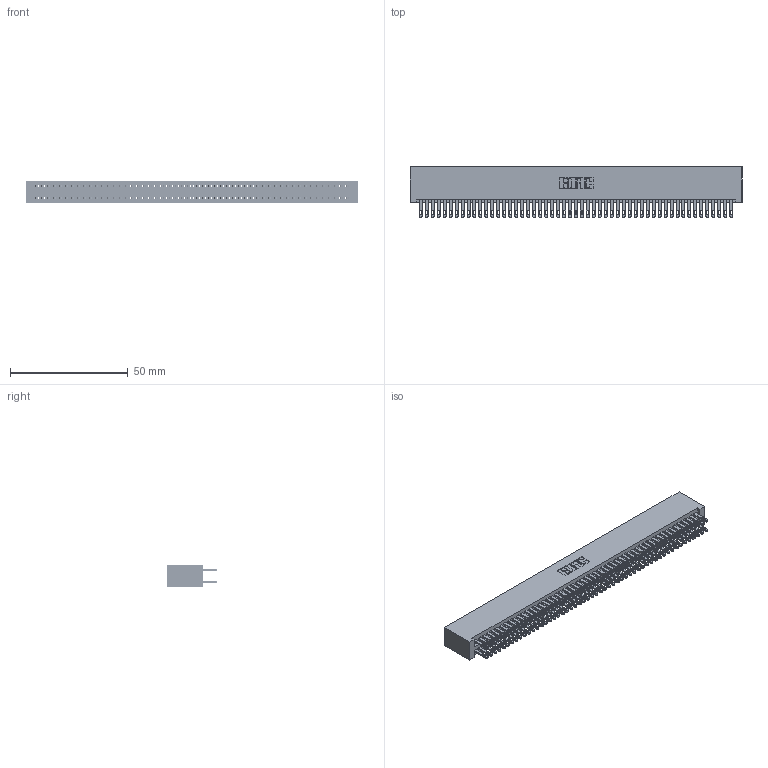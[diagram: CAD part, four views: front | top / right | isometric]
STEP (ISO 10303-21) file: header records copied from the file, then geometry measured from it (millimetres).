
FILE_DESCRIPTION (( 'STEP AP203' ), '1' );
FILE_NAME ('345-106-500-201.STEP', '2019-11-03T13:57:22', ( '' ), ( '' ), 'SwSTEP 2.0', 'SolidWorks 2016', '' );
FILE_SCHEMA (( 'CONFIG_CONTROL_DESIGN' ));
Length unit declared in the file: inch
Products named in the file (3): 345-106-500-201; 345 Part_No Mounting Lugs; 345-292-001_345-293-100
Assembly tree (107 placements, depth 2):
  345-106-500-201
    345 Part_No Mounting Lugs
    345-292-001_345-293-100  x106
Bounding box: 141.22 x 21.51 x 9.4 mm (x, y, z)
Volume: 14760.6 mm3; surface area: 23416.1 mm2
Topology: 107 solids, 107 shells, 4994 faces, 15263 edges, 10174 vertices
Faces by surface type: plane 2938, cylinder 2056
Entity records: 39757 total; most frequent: CARTESIAN_POINT 6652, ORIENTED_EDGE 6586, DIRECTION 5849, EDGE_CURVE 3293, VECTOR 2953, LINE 2953, VERTEX_POINT 2194, AXIS2_PLACEMENT_3D 1448
